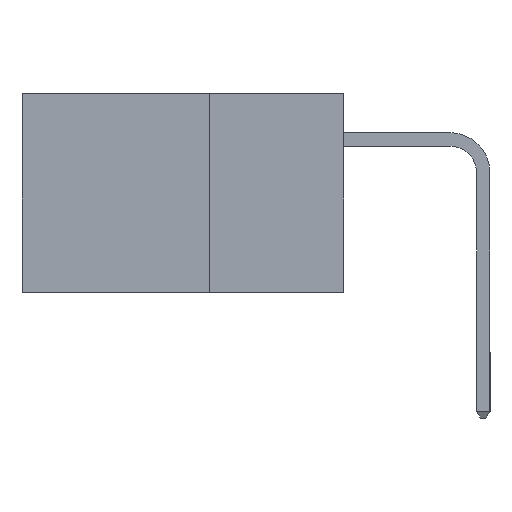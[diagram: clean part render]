
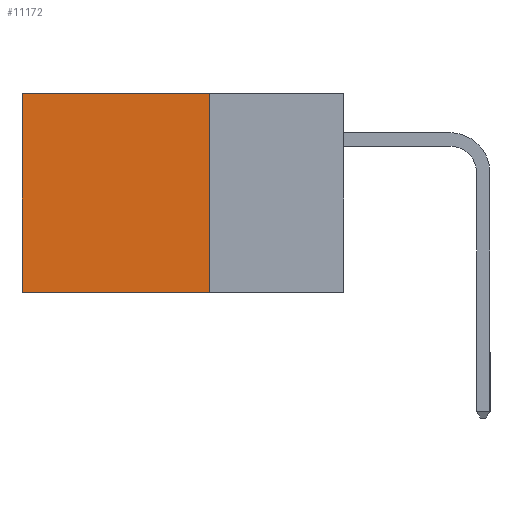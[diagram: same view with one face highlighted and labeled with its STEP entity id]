
A CAD part, left-side view. The second image highlights one B-rep face of the part: STEP entity #11172.
In plain terms, the highlighted planar face has unit normal (-1, 0, 0).
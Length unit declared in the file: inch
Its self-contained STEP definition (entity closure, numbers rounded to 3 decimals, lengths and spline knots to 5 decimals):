
#200 = ORIENTED_EDGE ( 'NONE', *, *, #13577, .F. ) ;
#628 = VERTEX_POINT ( 'NONE', #14475 ) ;
#974 = VERTEX_POINT ( 'NONE', #18313 ) ;
#1101 = VERTEX_POINT ( 'NONE', #10312 ) ;
#1957 = LINE ( 'NONE', #3589, #18989 ) ;
#3504 = ORIENTED_EDGE ( 'NONE', *, *, #5535, .T. ) ;
#3589 = CARTESIAN_POINT ( 'NONE',  ( 0.2615, 0.6, -0.37 ) ) ;
#4219 = CARTESIAN_POINT ( 'NONE',  ( 0.2615, 0.25, 0. ) ) ;
#5457 = VECTOR ( 'NONE', #18764, 39.37008 ) ;
#5535 = EDGE_CURVE ( 'NONE', #974, #1101, #1957, .T. ) ;
#5773 = DIRECTION ( 'NONE',  ( 0., 1., 0. ) ) ;
#5867 = LINE ( 'NONE', #14638, #6615 ) ;
#6247 = EDGE_CURVE ( 'NONE', #628, #974, #14722, .T. ) ;
#6615 = VECTOR ( 'NONE', #5773, 39.37008 ) ;
#6855 = ORIENTED_EDGE ( 'NONE', *, *, #13652, .F. ) ;
#8302 = EDGE_LOOP ( 'NONE', ( #3504, #6855, #200, #12950 ) ) ;
#8521 = PLANE ( 'NONE',  #16369 ) ;
#8618 = DIRECTION ( 'NONE',  ( 1., 0., 0. ) ) ;
#10312 = CARTESIAN_POINT ( 'NONE',  ( 0.2615, 0.6, -0.37 ) ) ;
#11172 = ADVANCED_FACE ( 'NONE', ( #17107 ), #8521, .F. ) ;
#12426 = CARTESIAN_POINT ( 'NONE',  ( 0.2615, 0.25, -0.37 ) ) ;
#12704 = LINE ( 'NONE', #12426, #16461 ) ;
#12950 = ORIENTED_EDGE ( 'NONE', *, *, #6247, .T. ) ;
#13058 = CARTESIAN_POINT ( 'NONE',  ( 0.2615, 0.25, -0.37 ) ) ;
#13577 = EDGE_CURVE ( 'NONE', #628, #18070, #12704, .T. ) ;
#13652 = EDGE_CURVE ( 'NONE', #18070, #1101, #5867, .T. ) ;
#14475 = CARTESIAN_POINT ( 'NONE',  ( 0.2615, 0.25, 0. ) ) ;
#14599 = DIRECTION ( 'NONE',  ( 0., 0., -1. ) ) ;
#14638 = CARTESIAN_POINT ( 'NONE',  ( 0.2615, 0.25, -0.37 ) ) ;
#14722 = LINE ( 'NONE', #4219, #5457 ) ;
#14951 = DIRECTION ( 'NONE',  ( 0., 0., -1. ) ) ;
#15413 = DIRECTION ( 'NONE',  ( 0., 0., -1. ) ) ;
#16357 = CARTESIAN_POINT ( 'NONE',  ( 0.2615, 0.25, -0.37 ) ) ;
#16369 = AXIS2_PLACEMENT_3D ( 'NONE', #13058, #8618, #14599 ) ;
#16461 = VECTOR ( 'NONE', #15413, 39.37008 ) ;
#17107 = FACE_OUTER_BOUND ( 'NONE', #8302, .T. ) ;
#18070 = VERTEX_POINT ( 'NONE', #16357 ) ;
#18313 = CARTESIAN_POINT ( 'NONE',  ( 0.2615, 0.6, 0. ) ) ;
#18764 = DIRECTION ( 'NONE',  ( 0., 1., 0. ) ) ;
#18989 = VECTOR ( 'NONE', #14951, 39.37008 ) ;
